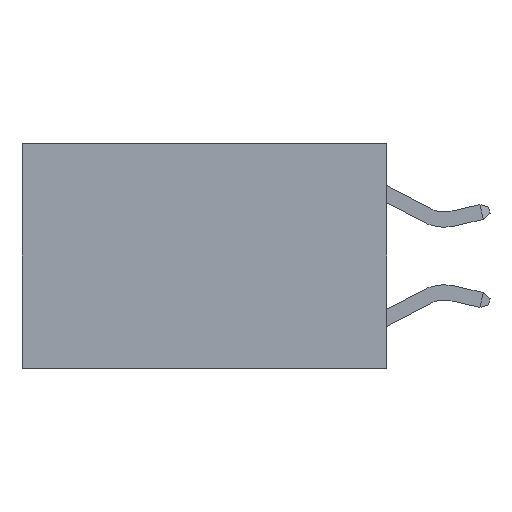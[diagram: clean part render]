
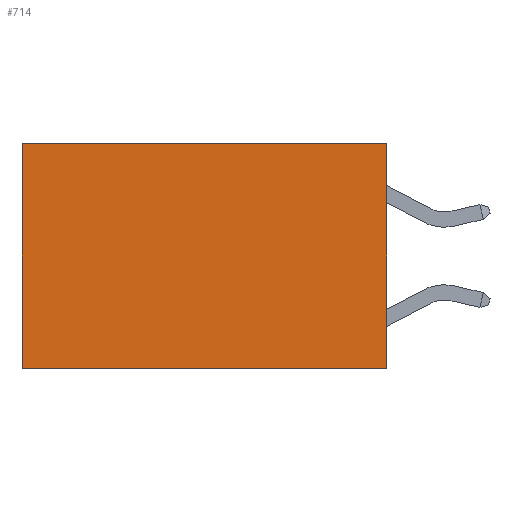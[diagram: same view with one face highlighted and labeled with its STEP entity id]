
A CAD part, left-side view. The second image highlights one B-rep face of the part: STEP entity #714.
In plain terms, the highlighted planar face has unit normal (-1, 0, 0).
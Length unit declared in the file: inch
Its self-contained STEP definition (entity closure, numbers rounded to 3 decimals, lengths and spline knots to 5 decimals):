
#549 = VECTOR ( 'NONE', #3159, 39.37008 ) ;
#714 = ADVANCED_FACE ( 'NONE', ( #865 ), #2063, .F. ) ;
#865 = FACE_OUTER_BOUND ( 'NONE', #12260, .T. ) ;
#1041 = EDGE_CURVE ( 'NONE', #4664, #14640, #8898, .T. ) ;
#1151 = VECTOR ( 'NONE', #2518, 39.37008 ) ;
#2063 = PLANE ( 'NONE',  #5578 ) ;
#2285 = CARTESIAN_POINT ( 'NONE',  ( 0.2625, 0.6, -0.37 ) ) ;
#2518 = DIRECTION ( 'NONE',  ( 0., 0., -1. ) ) ;
#2818 = VECTOR ( 'NONE', #4868, 39.37008 ) ;
#3087 = ORIENTED_EDGE ( 'NONE', *, *, #13462, .F. ) ;
#3159 = DIRECTION ( 'NONE',  ( 0., 0., -1. ) ) ;
#3485 = VERTEX_POINT ( 'NONE', #6320 ) ;
#4664 = VERTEX_POINT ( 'NONE', #13965 ) ;
#4868 = DIRECTION ( 'NONE',  ( 0., 1., 0. ) ) ;
#4960 = VERTEX_POINT ( 'NONE', #7035 ) ;
#5169 = ORIENTED_EDGE ( 'NONE', *, *, #12987, .F. ) ;
#5578 = AXIS2_PLACEMENT_3D ( 'NONE', #11569, #5803, #8012 ) ;
#5803 = DIRECTION ( 'NONE',  ( 1., 0., 0. ) ) ;
#6196 = LINE ( 'NONE', #10716, #2818 ) ;
#6320 = CARTESIAN_POINT ( 'NONE',  ( 0.2625, 0., 0. ) ) ;
#7035 = CARTESIAN_POINT ( 'NONE',  ( 0.2625, 0., -0.37 ) ) ;
#7883 = LINE ( 'NONE', #11663, #10839 ) ;
#7931 = EDGE_CURVE ( 'NONE', #3485, #4664, #7883, .T. ) ;
#8012 = DIRECTION ( 'NONE',  ( 0., 0., -1. ) ) ;
#8118 = LINE ( 'NONE', #12725, #1151 ) ;
#8898 = LINE ( 'NONE', #13577, #549 ) ;
#10716 = CARTESIAN_POINT ( 'NONE',  ( 0.2625, 0., -0.37 ) ) ;
#10839 = VECTOR ( 'NONE', #11450, 39.37008 ) ;
#11450 = DIRECTION ( 'NONE',  ( 0., 1., 0. ) ) ;
#11569 = CARTESIAN_POINT ( 'NONE',  ( 0.2625, 0., 0. ) ) ;
#11663 = CARTESIAN_POINT ( 'NONE',  ( 0.2625, 0., 0. ) ) ;
#12260 = EDGE_LOOP ( 'NONE', ( #13881, #3087, #5169, #12305 ) ) ;
#12305 = ORIENTED_EDGE ( 'NONE', *, *, #7931, .T. ) ;
#12725 = CARTESIAN_POINT ( 'NONE',  ( 0.2625, 0., 0. ) ) ;
#12987 = EDGE_CURVE ( 'NONE', #3485, #4960, #8118, .T. ) ;
#13462 = EDGE_CURVE ( 'NONE', #4960, #14640, #6196, .T. ) ;
#13577 = CARTESIAN_POINT ( 'NONE',  ( 0.2625, 0.6, 0. ) ) ;
#13881 = ORIENTED_EDGE ( 'NONE', *, *, #1041, .T. ) ;
#13965 = CARTESIAN_POINT ( 'NONE',  ( 0.2625, 0.6, 0. ) ) ;
#14640 = VERTEX_POINT ( 'NONE', #2285 ) ;
